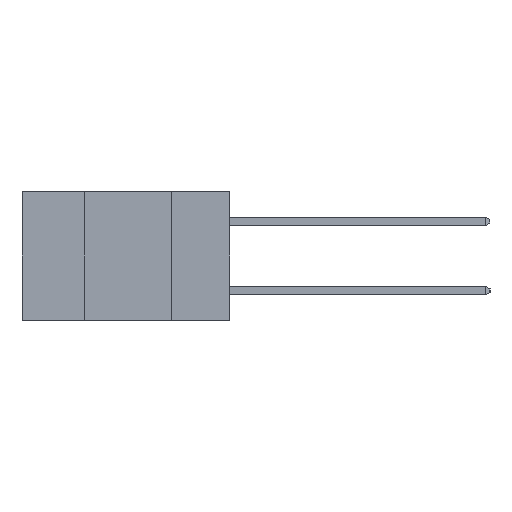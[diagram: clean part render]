
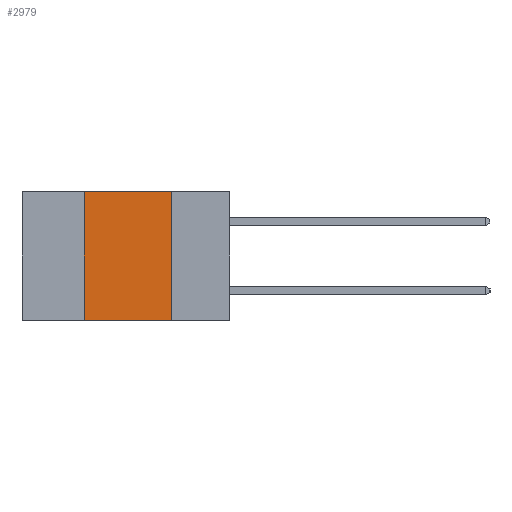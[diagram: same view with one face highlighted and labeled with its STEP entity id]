
A CAD part, left-side view. The second image highlights one B-rep face of the part: STEP entity #2979.
In plain terms, the highlighted planar face has unit normal (-1, 0, 0).
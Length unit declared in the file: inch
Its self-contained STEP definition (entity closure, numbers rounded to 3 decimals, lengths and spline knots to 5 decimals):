
#276 = VERTEX_POINT ( 'NONE', #5098 ) ;
#286 = FACE_OUTER_BOUND ( 'NONE', #8796, .T. ) ;
#815 = DIRECTION ( 'NONE',  ( 1., 0., 0. ) ) ;
#933 = ORIENTED_EDGE ( 'NONE', *, *, #2401, .T. ) ;
#1135 = LINE ( 'NONE', #13527, #7786 ) ;
#2401 = EDGE_CURVE ( 'NONE', #276, #11309, #5528, .T. ) ;
#2837 = AXIS2_PLACEMENT_3D ( 'NONE', #12042, #815, #12824 ) ;
#2979 = ADVANCED_FACE ( 'NONE', ( #286 ), #9698, .F. ) ;
#5098 = CARTESIAN_POINT ( 'NONE',  ( 0., 0.42, -0.37 ) ) ;
#5528 = LINE ( 'NONE', #9288, #15503 ) ;
#5648 = CARTESIAN_POINT ( 'NONE',  ( 0., 0.17, 0. ) ) ;
#6758 = ORIENTED_EDGE ( 'NONE', *, *, #13734, .F. ) ;
#7173 = ORIENTED_EDGE ( 'NONE', *, *, #10814, .F. ) ;
#7786 = VECTOR ( 'NONE', #14793, 39.37008 ) ;
#8796 = EDGE_LOOP ( 'NONE', ( #6758, #7173, #14522, #933 ) ) ;
#9288 = CARTESIAN_POINT ( 'NONE',  ( 0., 0.6, -0.37 ) ) ;
#9569 = VECTOR ( 'NONE', #11240, 39.37008 ) ;
#9698 = PLANE ( 'NONE',  #2837 ) ;
#9906 = CARTESIAN_POINT ( 'NONE',  ( 0., 0.42, -0.37 ) ) ;
#10216 = VERTEX_POINT ( 'NONE', #5648 ) ;
#10643 = DIRECTION ( 'NONE',  ( 0., -1., 0. ) ) ;
#10814 = EDGE_CURVE ( 'NONE', #13424, #10216, #14218, .T. ) ;
#11240 = DIRECTION ( 'NONE',  ( 0., 0., 1. ) ) ;
#11309 = VERTEX_POINT ( 'NONE', #12586 ) ;
#11974 = CARTESIAN_POINT ( 'NONE',  ( 0., 0.6, 0. ) ) ;
#12042 = CARTESIAN_POINT ( 'NONE',  ( 0., 0.6, 0. ) ) ;
#12586 = CARTESIAN_POINT ( 'NONE',  ( 0., 0.17, -0.37 ) ) ;
#12824 = DIRECTION ( 'NONE',  ( 0., 0., -1. ) ) ;
#13252 = DIRECTION ( 'NONE',  ( 0., -1., 0. ) ) ;
#13424 = VERTEX_POINT ( 'NONE', #15413 ) ;
#13527 = CARTESIAN_POINT ( 'NONE',  ( 0., 0.17, -0.37 ) ) ;
#13734 = EDGE_CURVE ( 'NONE', #10216, #11309, #1135, .T. ) ;
#13822 = VECTOR ( 'NONE', #13252, 39.37008 ) ;
#14218 = LINE ( 'NONE', #11974, #13822 ) ;
#14522 = ORIENTED_EDGE ( 'NONE', *, *, #15109, .F. ) ;
#14793 = DIRECTION ( 'NONE',  ( 0., 0., -1. ) ) ;
#15109 = EDGE_CURVE ( 'NONE', #276, #13424, #16417, .T. ) ;
#15413 = CARTESIAN_POINT ( 'NONE',  ( 0., 0.42, 0. ) ) ;
#15503 = VECTOR ( 'NONE', #10643, 39.37008 ) ;
#16417 = LINE ( 'NONE', #9906, #9569 ) ;
